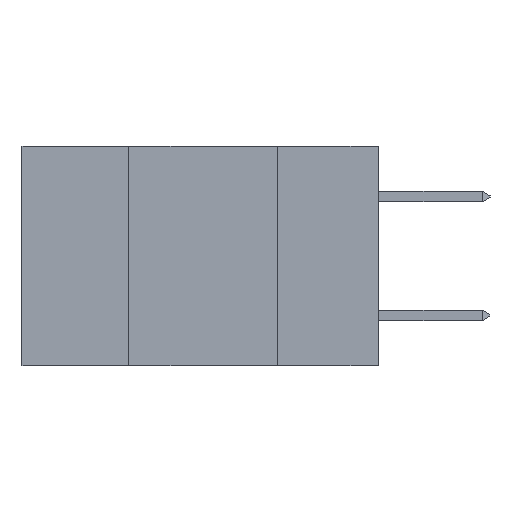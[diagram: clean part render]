
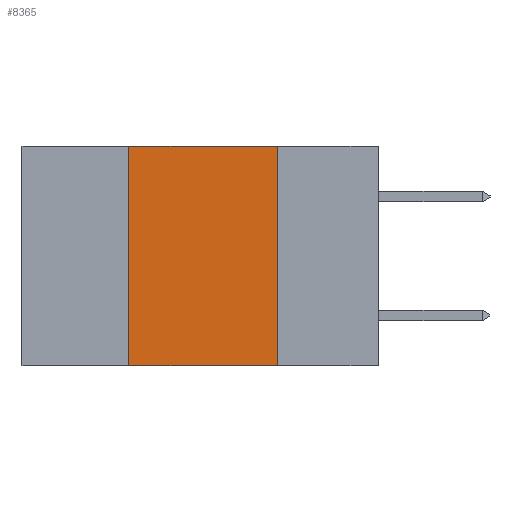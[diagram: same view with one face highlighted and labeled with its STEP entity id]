
A CAD part, left-side view. The second image highlights one B-rep face of the part: STEP entity #8365.
In plain terms, the highlighted planar face has unit normal (-1, 0, 0).
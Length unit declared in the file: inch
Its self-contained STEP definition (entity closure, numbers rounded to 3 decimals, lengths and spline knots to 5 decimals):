
#1195 = VERTEX_POINT ( 'NONE', #6057 ) ;
#1287 = CARTESIAN_POINT ( 'NONE',  ( 0., 0.6, 0. ) ) ;
#1764 = EDGE_CURVE ( 'NONE', #4695, #7050, #6938, .T. ) ;
#1989 = CARTESIAN_POINT ( 'NONE',  ( 0., 0.6, -0.37 ) ) ;
#2024 = PLANE ( 'NONE',  #4816 ) ;
#2025 = DIRECTION ( 'NONE',  ( 0., -1., 0. ) ) ;
#2771 = VECTOR ( 'NONE', #7531, 39.37008 ) ;
#2841 = DIRECTION ( 'NONE',  ( 0., 0., -1. ) ) ;
#3101 = ORIENTED_EDGE ( 'NONE', *, *, #5454, .T. ) ;
#3629 = VERTEX_POINT ( 'NONE', #7470 ) ;
#3984 = ORIENTED_EDGE ( 'NONE', *, *, #6427, .F. ) ;
#4272 = EDGE_CURVE ( 'NONE', #7050, #3629, #4710, .T. ) ;
#4299 = LINE ( 'NONE', #1989, #8417 ) ;
#4695 = VERTEX_POINT ( 'NONE', #9236 ) ;
#4710 = LINE ( 'NONE', #10149, #6974 ) ;
#4816 = AXIS2_PLACEMENT_3D ( 'NONE', #8286, #7507, #2841 ) ;
#5149 = ORIENTED_EDGE ( 'NONE', *, *, #1764, .F. ) ;
#5350 = CARTESIAN_POINT ( 'NONE',  ( 0., 0.42, 0. ) ) ;
#5377 = LINE ( 'NONE', #5350, #9242 ) ;
#5454 = EDGE_CURVE ( 'NONE', #1195, #3629, #4299, .T. ) ;
#5455 = FACE_OUTER_BOUND ( 'NONE', #5937, .T. ) ;
#5704 = DIRECTION ( 'NONE',  ( 0., 0., 1. ) ) ;
#5765 = DIRECTION ( 'NONE',  ( 0., 0., -1. ) ) ;
#5937 = EDGE_LOOP ( 'NONE', ( #6012, #5149, #3984, #3101 ) ) ;
#6012 = ORIENTED_EDGE ( 'NONE', *, *, #4272, .F. ) ;
#6057 = CARTESIAN_POINT ( 'NONE',  ( 0., 0.42, -0.37 ) ) ;
#6427 = EDGE_CURVE ( 'NONE', #1195, #4695, #5377, .T. ) ;
#6938 = LINE ( 'NONE', #1287, #2771 ) ;
#6974 = VECTOR ( 'NONE', #5765, 39.37008 ) ;
#7050 = VERTEX_POINT ( 'NONE', #9635 ) ;
#7470 = CARTESIAN_POINT ( 'NONE',  ( 0., 0.17, -0.37 ) ) ;
#7507 = DIRECTION ( 'NONE',  ( 1., 0., 0. ) ) ;
#7531 = DIRECTION ( 'NONE',  ( 0., -1., 0. ) ) ;
#8286 = CARTESIAN_POINT ( 'NONE',  ( 0., 0.6, 0. ) ) ;
#8365 = ADVANCED_FACE ( 'NONE', ( #5455 ), #2024, .F. ) ;
#8417 = VECTOR ( 'NONE', #2025, 39.37008 ) ;
#9236 = CARTESIAN_POINT ( 'NONE',  ( 0., 0.42, 0. ) ) ;
#9242 = VECTOR ( 'NONE', #5704, 39.37008 ) ;
#9635 = CARTESIAN_POINT ( 'NONE',  ( 0., 0.17, 0. ) ) ;
#10149 = CARTESIAN_POINT ( 'NONE',  ( 0., 0.17, 0. ) ) ;
